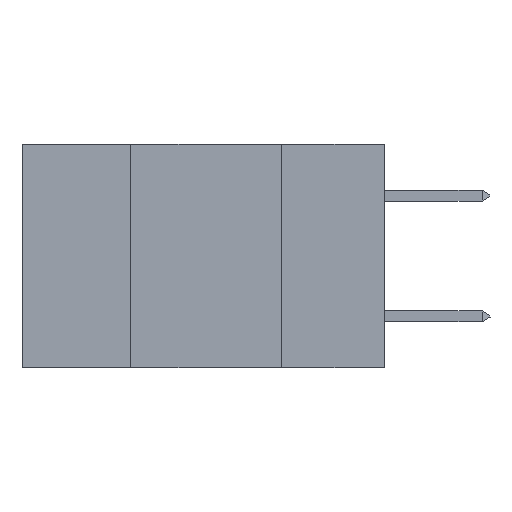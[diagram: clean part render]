
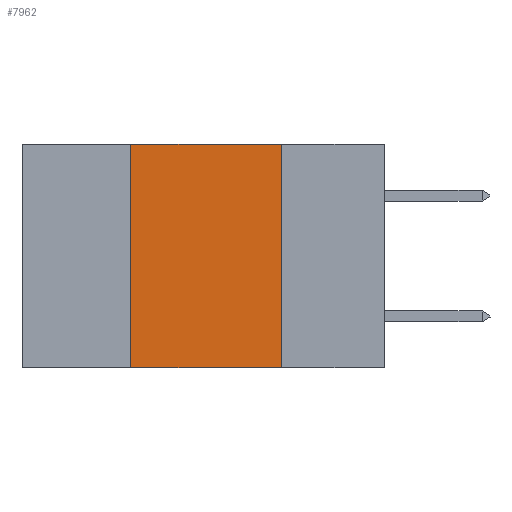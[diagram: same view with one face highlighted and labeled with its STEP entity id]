
A CAD part, left-side view. The second image highlights one B-rep face of the part: STEP entity #7962.
In plain terms, the highlighted planar face has unit normal (-1, 0, 0).
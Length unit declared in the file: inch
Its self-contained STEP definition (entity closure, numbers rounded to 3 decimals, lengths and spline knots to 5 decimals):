
#684 = CARTESIAN_POINT ( 'NONE',  ( 0., 0.6, 0. ) ) ;
#1843 = VECTOR ( 'NONE', #9529, 39.37008 ) ;
#2023 = CARTESIAN_POINT ( 'NONE',  ( 0., 0.6, 0. ) ) ;
#2121 = VECTOR ( 'NONE', #14205, 39.37008 ) ;
#2709 = ORIENTED_EDGE ( 'NONE', *, *, #8204, .F. ) ;
#3179 = LINE ( 'NONE', #4456, #7186 ) ;
#3331 = VERTEX_POINT ( 'NONE', #5501 ) ;
#3802 = VERTEX_POINT ( 'NONE', #18950 ) ;
#4325 = CARTESIAN_POINT ( 'NONE',  ( 0., 0.6, -0.37 ) ) ;
#4456 = CARTESIAN_POINT ( 'NONE',  ( 0., 0.17, 0. ) ) ;
#4478 = EDGE_LOOP ( 'NONE', ( #2709, #20451, #14426, #14842 ) ) ;
#5501 = CARTESIAN_POINT ( 'NONE',  ( 0., 0.42, 0. ) ) ;
#5555 = PLANE ( 'NONE',  #15180 ) ;
#5948 = LINE ( 'NONE', #19652, #1843 ) ;
#6194 = DIRECTION ( 'NONE',  ( 0., 0., -1. ) ) ;
#6672 = EDGE_CURVE ( 'NONE', #12686, #3331, #5948, .T. ) ;
#7186 = VECTOR ( 'NONE', #6194, 39.37008 ) ;
#7537 = EDGE_CURVE ( 'NONE', #3331, #19296, #11169, .T. ) ;
#7962 = ADVANCED_FACE ( 'NONE', ( #15083 ), #5555, .F. ) ;
#8204 = EDGE_CURVE ( 'NONE', #19296, #3802, #3179, .T. ) ;
#8906 = DIRECTION ( 'NONE',  ( 0., 0., -1. ) ) ;
#9529 = DIRECTION ( 'NONE',  ( 0., 0., 1. ) ) ;
#11169 = LINE ( 'NONE', #684, #2121 ) ;
#11731 = EDGE_CURVE ( 'NONE', #12686, #3802, #19535, .T. ) ;
#12319 = CARTESIAN_POINT ( 'NONE',  ( 0., 0.42, -0.37 ) ) ;
#12686 = VERTEX_POINT ( 'NONE', #12319 ) ;
#14205 = DIRECTION ( 'NONE',  ( 0., -1., 0. ) ) ;
#14426 = ORIENTED_EDGE ( 'NONE', *, *, #6672, .F. ) ;
#14842 = ORIENTED_EDGE ( 'NONE', *, *, #11731, .T. ) ;
#15032 = VECTOR ( 'NONE', #21196, 39.37008 ) ;
#15083 = FACE_OUTER_BOUND ( 'NONE', #4478, .T. ) ;
#15180 = AXIS2_PLACEMENT_3D ( 'NONE', #2023, #19000, #8906 ) ;
#17717 = CARTESIAN_POINT ( 'NONE',  ( 0., 0.17, 0. ) ) ;
#18950 = CARTESIAN_POINT ( 'NONE',  ( 0., 0.17, -0.37 ) ) ;
#19000 = DIRECTION ( 'NONE',  ( 1., 0., 0. ) ) ;
#19296 = VERTEX_POINT ( 'NONE', #17717 ) ;
#19535 = LINE ( 'NONE', #4325, #15032 ) ;
#19652 = CARTESIAN_POINT ( 'NONE',  ( 0., 0.42, 0. ) ) ;
#20451 = ORIENTED_EDGE ( 'NONE', *, *, #7537, .F. ) ;
#21196 = DIRECTION ( 'NONE',  ( 0., -1., 0. ) ) ;
